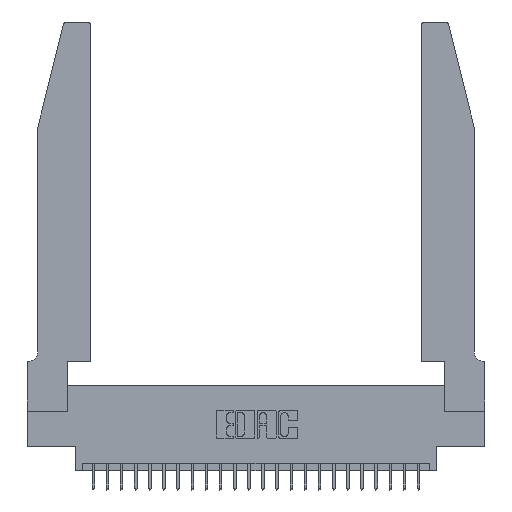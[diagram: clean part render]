
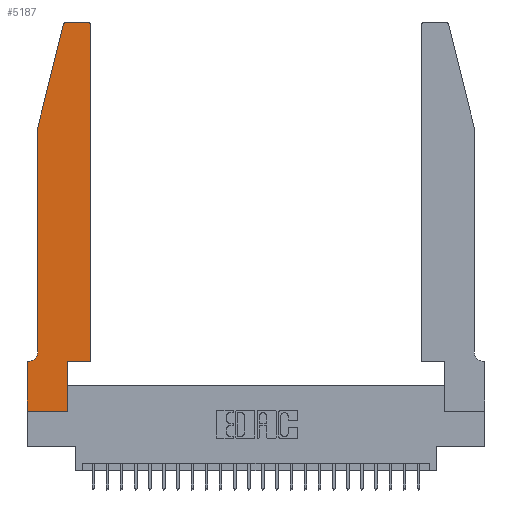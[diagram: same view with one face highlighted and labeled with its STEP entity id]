
A CAD part, top view. The second image highlights one B-rep face of the part: STEP entity #5187.
In plain terms, the highlighted planar face has unit normal (0, 0, 1).
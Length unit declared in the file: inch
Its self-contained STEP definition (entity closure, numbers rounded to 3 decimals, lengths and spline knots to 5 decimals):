
#40 = DIRECTION ( 'NONE',  ( 0., 0., 1. ) ) ;
#273 = VERTEX_POINT ( 'NONE', #12476 ) ;
#430 = FACE_OUTER_BOUND ( 'NONE', #9376, .T. ) ;
#702 = EDGE_CURVE ( 'NONE', #23482, #24877, #26212, .T. ) ;
#710 = AXIS2_PLACEMENT_3D ( 'NONE', #16798, #40, #14797 ) ;
#744 = DIRECTION ( 'NONE',  ( 1., 0., 0. ) ) ;
#998 = LINE ( 'NONE', #2768, #2807 ) ;
#1130 = VERTEX_POINT ( 'NONE', #2271 ) ;
#1703 = CIRCLE ( 'NONE', #18743, 0.03 ) ;
#1791 = ORIENTED_EDGE ( 'NONE', *, *, #11645, .T. ) ;
#1938 = VECTOR ( 'NONE', #20949, 39.37008 ) ;
#1939 = ORIENTED_EDGE ( 'NONE', *, *, #21052, .T. ) ;
#1976 = AXIS2_PLACEMENT_3D ( 'NONE', #22544, #24760, #8958 ) ;
#2271 = CARTESIAN_POINT ( 'NONE',  ( 0., 0., 0.37 ) ) ;
#2301 = CARTESIAN_POINT ( 'NONE',  ( 0.0755, 2., 0.37 ) ) ;
#2768 = CARTESIAN_POINT ( 'NONE',  ( 0.4505, 0.35, 0.37 ) ) ;
#2807 = VECTOR ( 'NONE', #744, 39.37008 ) ;
#2933 = EDGE_CURVE ( 'NONE', #12587, #20261, #18262, .T. ) ;
#3554 = EDGE_CURVE ( 'NONE', #8740, #1130, #23531, .T. ) ;
#3626 = DIRECTION ( 'NONE',  ( -1., 0., 0. ) ) ;
#3715 = VERTEX_POINT ( 'NONE', #22214 ) ;
#3966 = CARTESIAN_POINT ( 'NONE',  ( 0.4205, 2.72, 0.37 ) ) ;
#4155 = VERTEX_POINT ( 'NONE', #7778 ) ;
#4266 = EDGE_CURVE ( 'NONE', #1130, #12587, #24485, .T. ) ;
#4971 = EDGE_CURVE ( 'NONE', #20261, #4155, #998, .T. ) ;
#5073 = ORIENTED_EDGE ( 'NONE', *, *, #11127, .T. ) ;
#5187 = ADVANCED_FACE ( 'NONE', ( #430 ), #16687, .T. ) ;
#5269 = CARTESIAN_POINT ( 'NONE',  ( 0.0755, 0.42, 0.37 ) ) ;
#5302 = VECTOR ( 'NONE', #5629, 39.37008 ) ;
#5342 = VECTOR ( 'NONE', #11585, 39.37008 ) ;
#5509 = CARTESIAN_POINT ( 'NONE',  ( 0.2605, 2.75, 0.37 ) ) ;
#5622 = LINE ( 'NONE', #9747, #8940 ) ;
#5629 = DIRECTION ( 'NONE',  ( 0., 1., 0. ) ) ;
#5707 = ORIENTED_EDGE ( 'NONE', *, *, #4971, .T. ) ;
#5956 = EDGE_CURVE ( 'NONE', #22804, #273, #16882, .T. ) ;
#6001 = CARTESIAN_POINT ( 'NONE',  ( 0.4205, 2.75, 0.37 ) ) ;
#6752 = DIRECTION ( 'NONE',  ( 0., 1., 0. ) ) ;
#6807 = VECTOR ( 'NONE', #6752, 39.37008 ) ;
#7413 = ORIENTED_EDGE ( 'NONE', *, *, #26226, .T. ) ;
#7778 = CARTESIAN_POINT ( 'NONE',  ( 0.4505, 0.35, 0.37 ) ) ;
#8170 = DIRECTION ( 'NONE',  ( 0., -1., 0. ) ) ;
#8274 = EDGE_CURVE ( 'NONE', #24877, #19228, #9314, .T. ) ;
#8740 = VERTEX_POINT ( 'NONE', #21105 ) ;
#8940 = VECTOR ( 'NONE', #24190, 39.37008 ) ;
#8958 = DIRECTION ( 'NONE',  ( 1., 0., 0. ) ) ;
#9314 = CIRCLE ( 'NONE', #24554, 0.07 ) ;
#9376 = EDGE_LOOP ( 'NONE', ( #7413, #16559, #5073, #13762, #18553, #1939, #21439, #9723, #14878, #5707, #1791, #16778 ) ) ;
#9723 = ORIENTED_EDGE ( 'NONE', *, *, #4266, .T. ) ;
#9747 = CARTESIAN_POINT ( 'NONE',  ( 0.0755, 2., 0.37 ) ) ;
#11024 = CARTESIAN_POINT ( 'NONE',  ( 0.4505, 0.35, 0.37 ) ) ;
#11127 = EDGE_CURVE ( 'NONE', #273, #23482, #5622, .T. ) ;
#11585 = DIRECTION ( 'NONE',  ( 0., -1., 0. ) ) ;
#11645 = EDGE_CURVE ( 'NONE', #4155, #3715, #23120, .T. ) ;
#12476 = CARTESIAN_POINT ( 'NONE',  ( 0.25487, 2.72718, 0.37 ) ) ;
#12587 = VERTEX_POINT ( 'NONE', #13185 ) ;
#13185 = CARTESIAN_POINT ( 'NONE',  ( 0.2865, 0., 0.37 ) ) ;
#13762 = ORIENTED_EDGE ( 'NONE', *, *, #702, .T. ) ;
#14566 = VECTOR ( 'NONE', #3626, 39.37008 ) ;
#14797 = DIRECTION ( 'NONE',  ( 1., 0., 0. ) ) ;
#14878 = ORIENTED_EDGE ( 'NONE', *, *, #2933, .T. ) ;
#15281 = CARTESIAN_POINT ( 'NONE',  ( 0.0055, 0.35, 0.37 ) ) ;
#15283 = DIRECTION ( 'NONE',  ( 0., 0., -1. ) ) ;
#15728 = CARTESIAN_POINT ( 'NONE',  ( 0.2865, 0.35, 0.37 ) ) ;
#16188 = DIRECTION ( 'NONE',  ( 0., 0., 1. ) ) ;
#16519 = VECTOR ( 'NONE', #19404, 39.37008 ) ;
#16559 = ORIENTED_EDGE ( 'NONE', *, *, #5956, .T. ) ;
#16677 = CARTESIAN_POINT ( 'NONE',  ( 0., 0., 0.37 ) ) ;
#16687 = PLANE ( 'NONE',  #1976 ) ;
#16778 = ORIENTED_EDGE ( 'NONE', *, *, #23322, .T. ) ;
#16798 = CARTESIAN_POINT ( 'NONE',  ( 0.284, 2.72, 0.37 ) ) ;
#16882 = CIRCLE ( 'NONE', #710, 0.03 ) ;
#17691 = CARTESIAN_POINT ( 'NONE',  ( 0., 0., 0.37 ) ) ;
#17699 = CARTESIAN_POINT ( 'NONE',  ( 0.0055, 0.42, 0.37 ) ) ;
#18262 = LINE ( 'NONE', #15728, #5302 ) ;
#18553 = ORIENTED_EDGE ( 'NONE', *, *, #8274, .T. ) ;
#18743 = AXIS2_PLACEMENT_3D ( 'NONE', #3966, #16188, #22716 ) ;
#19228 = VERTEX_POINT ( 'NONE', #15281 ) ;
#19404 = DIRECTION ( 'NONE',  ( -1., 0., 0. ) ) ;
#19793 = CARTESIAN_POINT ( 'NONE',  ( 0.0755, 2., 0.37 ) ) ;
#20261 = VERTEX_POINT ( 'NONE', #23840 ) ;
#20490 = VERTEX_POINT ( 'NONE', #6001 ) ;
#20949 = DIRECTION ( 'NONE',  ( 1., 0., 0. ) ) ;
#21052 = EDGE_CURVE ( 'NONE', #19228, #8740, #21515, .T. ) ;
#21105 = CARTESIAN_POINT ( 'NONE',  ( 0., 0.35, 0.37 ) ) ;
#21155 = VECTOR ( 'NONE', #8170, 39.37008 ) ;
#21439 = ORIENTED_EDGE ( 'NONE', *, *, #3554, .T. ) ;
#21515 = LINE ( 'NONE', #25590, #16519 ) ;
#22133 = LINE ( 'NONE', #5509, #14566 ) ;
#22214 = CARTESIAN_POINT ( 'NONE',  ( 0.4505, 2.72, 0.37 ) ) ;
#22544 = CARTESIAN_POINT ( 'NONE',  ( 0., 0.35, 0.37 ) ) ;
#22716 = DIRECTION ( 'NONE',  ( 1., 0., 0. ) ) ;
#22804 = VERTEX_POINT ( 'NONE', #23419 ) ;
#23120 = LINE ( 'NONE', #11024, #6807 ) ;
#23322 = EDGE_CURVE ( 'NONE', #3715, #20490, #1703, .T. ) ;
#23403 = DIRECTION ( 'NONE',  ( -1., 0., 0. ) ) ;
#23419 = CARTESIAN_POINT ( 'NONE',  ( 0.284, 2.75, 0.37 ) ) ;
#23482 = VERTEX_POINT ( 'NONE', #19793 ) ;
#23531 = LINE ( 'NONE', #17691, #5342 ) ;
#23840 = CARTESIAN_POINT ( 'NONE',  ( 0.2865, 0.35, 0.37 ) ) ;
#24190 = DIRECTION ( 'NONE',  ( -0.239, -0.971, 0. ) ) ;
#24485 = LINE ( 'NONE', #16677, #1938 ) ;
#24554 = AXIS2_PLACEMENT_3D ( 'NONE', #17699, #15283, #23403 ) ;
#24760 = DIRECTION ( 'NONE',  ( 0., 0., 1. ) ) ;
#24877 = VERTEX_POINT ( 'NONE', #5269 ) ;
#25590 = CARTESIAN_POINT ( 'NONE',  ( 0.0755, 0.35, 0.37 ) ) ;
#26212 = LINE ( 'NONE', #2301, #21155 ) ;
#26226 = EDGE_CURVE ( 'NONE', #20490, #22804, #22133, .T. ) ;
